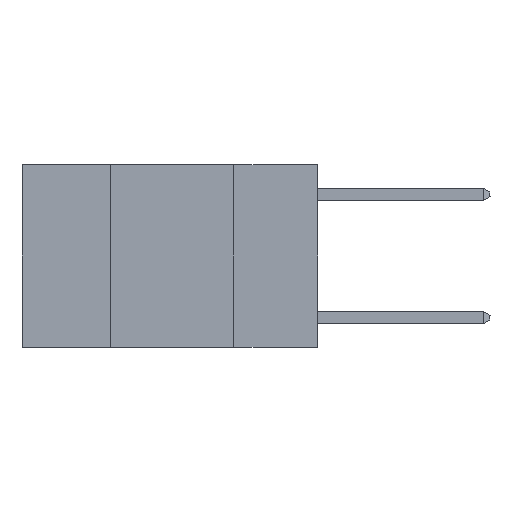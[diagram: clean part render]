
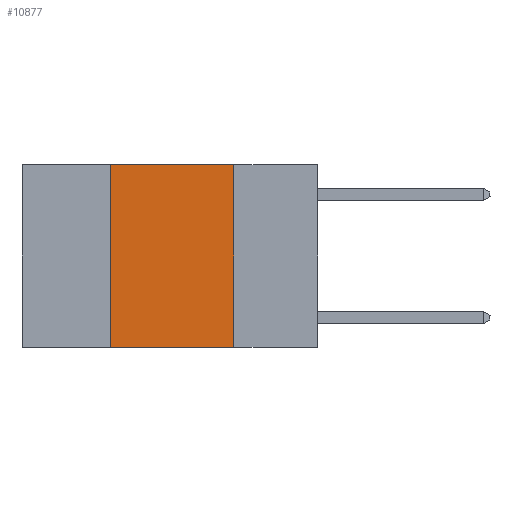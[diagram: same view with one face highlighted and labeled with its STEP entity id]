
A CAD part, left-side view. The second image highlights one B-rep face of the part: STEP entity #10877.
In plain terms, the highlighted planar face has unit normal (-1, 0, 0).
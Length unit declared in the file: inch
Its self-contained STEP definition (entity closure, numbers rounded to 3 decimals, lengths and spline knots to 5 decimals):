
#378 = VERTEX_POINT ( 'NONE', #22797 ) ;
#624 = CARTESIAN_POINT ( 'NONE',  ( 0., 0.6, -0.37 ) ) ;
#1848 = FACE_OUTER_BOUND ( 'NONE', #19369, .T. ) ;
#3007 = VERTEX_POINT ( 'NONE', #9011 ) ;
#3018 = DIRECTION ( 'NONE',  ( 0., -1., 0. ) ) ;
#3027 = CARTESIAN_POINT ( 'NONE',  ( 0., 0.17, -0.37 ) ) ;
#3442 = LINE ( 'NONE', #624, #15193 ) ;
#6192 = VECTOR ( 'NONE', #29880, 39.37008 ) ;
#6241 = ORIENTED_EDGE ( 'NONE', *, *, #29614, .F. ) ;
#6566 = DIRECTION ( 'NONE',  ( 0., -1., 0. ) ) ;
#6949 = VECTOR ( 'NONE', #6566, 39.37008 ) ;
#7506 = PLANE ( 'NONE',  #19775 ) ;
#8642 = VECTOR ( 'NONE', #28438, 39.37008 ) ;
#9011 = CARTESIAN_POINT ( 'NONE',  ( 0., 0.42, -0.37 ) ) ;
#10877 = ADVANCED_FACE ( 'NONE', ( #1848 ), #7506, .F. ) ;
#12186 = DIRECTION ( 'NONE',  ( 1., 0., 0. ) ) ;
#12384 = LINE ( 'NONE', #25342, #6192 ) ;
#12440 = ORIENTED_EDGE ( 'NONE', *, *, #22046, .T. ) ;
#15193 = VECTOR ( 'NONE', #3018, 39.37008 ) ;
#16318 = LINE ( 'NONE', #26174, #8642 ) ;
#16565 = VERTEX_POINT ( 'NONE', #18583 ) ;
#17205 = ORIENTED_EDGE ( 'NONE', *, *, #28111, .F. ) ;
#18583 = CARTESIAN_POINT ( 'NONE',  ( 0., 0.42, 0. ) ) ;
#18701 = EDGE_CURVE ( 'NONE', #16565, #378, #19398, .T. ) ;
#19369 = EDGE_LOOP ( 'NONE', ( #17205, #29425, #6241, #12440 ) ) ;
#19398 = LINE ( 'NONE', #25206, #6949 ) ;
#19775 = AXIS2_PLACEMENT_3D ( 'NONE', #26106, #12186, #28374 ) ;
#22046 = EDGE_CURVE ( 'NONE', #3007, #27089, #3442, .T. ) ;
#22797 = CARTESIAN_POINT ( 'NONE',  ( 0., 0.17, 0. ) ) ;
#25206 = CARTESIAN_POINT ( 'NONE',  ( 0., 0.6, 0. ) ) ;
#25342 = CARTESIAN_POINT ( 'NONE',  ( 0., 0.17, 0. ) ) ;
#26106 = CARTESIAN_POINT ( 'NONE',  ( 0., 0.6, 0. ) ) ;
#26174 = CARTESIAN_POINT ( 'NONE',  ( 0., 0.42, 0. ) ) ;
#27089 = VERTEX_POINT ( 'NONE', #3027 ) ;
#28111 = EDGE_CURVE ( 'NONE', #378, #27089, #12384, .T. ) ;
#28374 = DIRECTION ( 'NONE',  ( 0., 0., -1. ) ) ;
#28438 = DIRECTION ( 'NONE',  ( 0., 0., 1. ) ) ;
#29425 = ORIENTED_EDGE ( 'NONE', *, *, #18701, .F. ) ;
#29614 = EDGE_CURVE ( 'NONE', #3007, #16565, #16318, .T. ) ;
#29880 = DIRECTION ( 'NONE',  ( 0., 0., -1. ) ) ;
